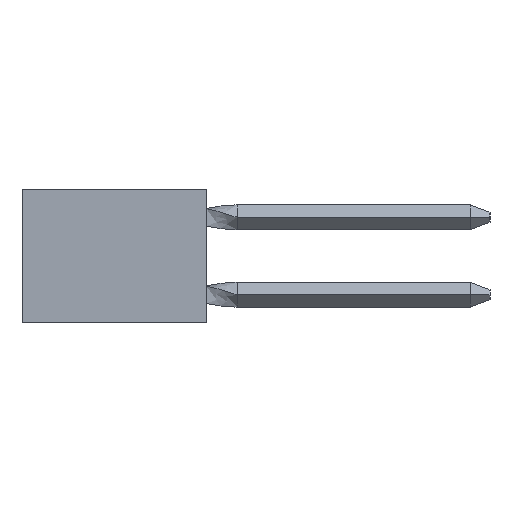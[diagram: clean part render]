
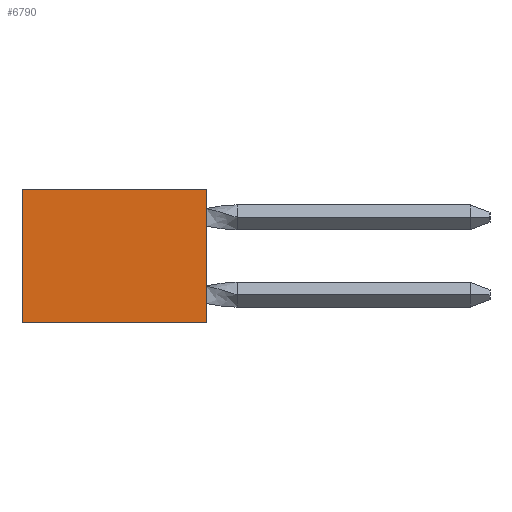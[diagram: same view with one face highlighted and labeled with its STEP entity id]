
A CAD part, left-side view. The second image highlights one B-rep face of the part: STEP entity #6790.
In plain terms, the highlighted planar face has unit normal (-1, 0, 0).
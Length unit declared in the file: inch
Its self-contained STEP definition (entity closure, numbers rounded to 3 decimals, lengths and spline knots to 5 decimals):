
#259 = EDGE_CURVE ( 'NONE', #13810, #10717, #538, .T. ) ;
#538 = LINE ( 'NONE', #7864, #14481 ) ;
#890 = EDGE_CURVE ( 'NONE', #10717, #14644, #15293, .T. ) ;
#1797 = CARTESIAN_POINT ( 'NONE',  ( 0.298, 0., -0.343 ) ) ;
#1855 = VECTOR ( 'NONE', #20477, 39.37008 ) ;
#1951 = EDGE_LOOP ( 'NONE', ( #21631, #2109, #21452, #19515 ) ) ;
#2109 = ORIENTED_EDGE ( 'NONE', *, *, #890, .T. ) ;
#2787 = LINE ( 'NONE', #18393, #17289 ) ;
#2796 = DIRECTION ( 'NONE',  ( 0., 0., 1. ) ) ;
#3268 = CARTESIAN_POINT ( 'NONE',  ( 0.298, -0.027, 0. ) ) ;
#4698 = VECTOR ( 'NONE', #6747, 39.37008 ) ;
#5941 = PLANE ( 'NONE',  #9164 ) ;
#6529 = CARTESIAN_POINT ( 'NONE',  ( 0.298, 0., 0. ) ) ;
#6747 = DIRECTION ( 'NONE',  ( 0., 0., -1. ) ) ;
#6790 = ADVANCED_FACE ( 'NONE', ( #17655 ), #5941, .F. ) ;
#6841 = CARTESIAN_POINT ( 'NONE',  ( 0.298, 0.473, -0.343 ) ) ;
#7864 = CARTESIAN_POINT ( 'NONE',  ( 0.298, 0., -0.343 ) ) ;
#8684 = EDGE_CURVE ( 'NONE', #13810, #20582, #2787, .T. ) ;
#9164 = AXIS2_PLACEMENT_3D ( 'NONE', #19921, #18079, #14552 ) ;
#10717 = VERTEX_POINT ( 'NONE', #6529 ) ;
#12375 = LINE ( 'NONE', #13885, #4698 ) ;
#12482 = EDGE_CURVE ( 'NONE', #14644, #20582, #12375, .T. ) ;
#13183 = DIRECTION ( 'NONE',  ( 0., 1., 0. ) ) ;
#13810 = VERTEX_POINT ( 'NONE', #1797 ) ;
#13885 = CARTESIAN_POINT ( 'NONE',  ( 0.298, 0.473, 0. ) ) ;
#14481 = VECTOR ( 'NONE', #2796, 39.37008 ) ;
#14552 = DIRECTION ( 'NONE',  ( 0., 0., -1. ) ) ;
#14644 = VERTEX_POINT ( 'NONE', #20107 ) ;
#15293 = LINE ( 'NONE', #3268, #1855 ) ;
#17289 = VECTOR ( 'NONE', #13183, 39.37008 ) ;
#17655 = FACE_OUTER_BOUND ( 'NONE', #1951, .T. ) ;
#18079 = DIRECTION ( 'NONE',  ( 1., 0., 0. ) ) ;
#18393 = CARTESIAN_POINT ( 'NONE',  ( 0.298, 0.473, -0.343 ) ) ;
#19515 = ORIENTED_EDGE ( 'NONE', *, *, #8684, .F. ) ;
#19921 = CARTESIAN_POINT ( 'NONE',  ( 0.298, -0.027, 0. ) ) ;
#20107 = CARTESIAN_POINT ( 'NONE',  ( 0.298, 0.473, 0. ) ) ;
#20477 = DIRECTION ( 'NONE',  ( 0., 1., 0. ) ) ;
#20582 = VERTEX_POINT ( 'NONE', #6841 ) ;
#21452 = ORIENTED_EDGE ( 'NONE', *, *, #12482, .T. ) ;
#21631 = ORIENTED_EDGE ( 'NONE', *, *, #259, .T. ) ;
